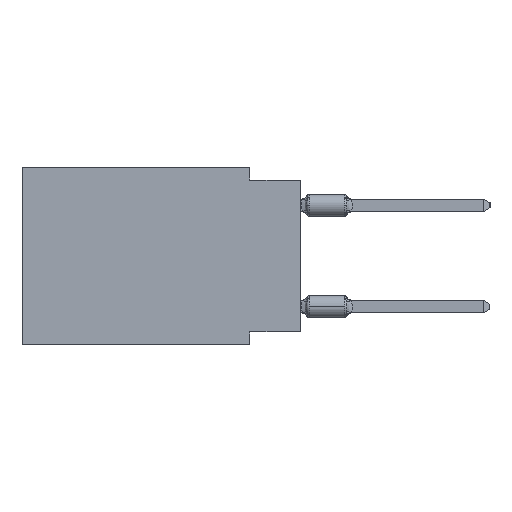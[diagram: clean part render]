
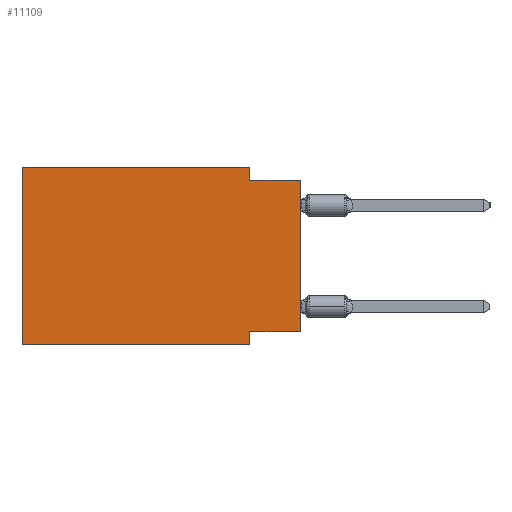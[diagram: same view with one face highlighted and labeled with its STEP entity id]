
A CAD part, left-side view. The second image highlights one B-rep face of the part: STEP entity #11109.
In plain terms, the highlighted planar face has unit normal (-1, 0, 0).
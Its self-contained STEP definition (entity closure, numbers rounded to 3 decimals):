
#362 = EDGE_CURVE ( 'NONE', #3799, #5954, #26076, .T. ) ;
#627 = ORIENTED_EDGE ( 'NONE', *, *, #13560, .T. ) ;
#1425 = LINE ( 'NONE', #3685, #17631 ) ;
#2826 = ORIENTED_EDGE ( 'NONE', *, *, #362, .F. ) ;
#3096 = EDGE_CURVE ( 'NONE', #16999, #22107, #26939, .T. ) ;
#3187 = EDGE_CURVE ( 'NONE', #3863, #16999, #23690, .T. ) ;
#3685 = CARTESIAN_POINT ( 'NONE',  ( 0., 13.97, -8.89 ) ) ;
#3799 = VERTEX_POINT ( 'NONE', #5236 ) ;
#3835 = VECTOR ( 'NONE', #4598, 1000. ) ;
#3863 = VERTEX_POINT ( 'NONE', #5098 ) ;
#4058 = CARTESIAN_POINT ( 'NONE',  ( 0., 13.97, 0. ) ) ;
#4166 = CARTESIAN_POINT ( 'NONE',  ( 0., 0., -8.255 ) ) ;
#4598 = DIRECTION ( 'NONE',  ( 0., 0., 1. ) ) ;
#4613 = VECTOR ( 'NONE', #23969, 1000. ) ;
#4740 = CARTESIAN_POINT ( 'NONE',  ( 0., 0., 0. ) ) ;
#5098 = CARTESIAN_POINT ( 'NONE',  ( 0., 0., -8.255 ) ) ;
#5126 = CARTESIAN_POINT ( 'NONE',  ( 0., 2.54, -8.255 ) ) ;
#5151 = EDGE_CURVE ( 'NONE', #5954, #16354, #18944, .T. ) ;
#5236 = CARTESIAN_POINT ( 'NONE',  ( 0., 2.54, 0. ) ) ;
#5716 = ORIENTED_EDGE ( 'NONE', *, *, #3187, .F. ) ;
#5859 = CARTESIAN_POINT ( 'NONE',  ( 0., 13.97, 0. ) ) ;
#5954 = VERTEX_POINT ( 'NONE', #16780 ) ;
#6368 = EDGE_CURVE ( 'NONE', #6394, #22107, #1425, .T. ) ;
#6394 = VERTEX_POINT ( 'NONE', #14779 ) ;
#6710 = VECTOR ( 'NONE', #27196, 1000. ) ;
#8221 = CARTESIAN_POINT ( 'NONE',  ( 0., 13.97, 0. ) ) ;
#8245 = VECTOR ( 'NONE', #16263, 1000. ) ;
#8878 = CARTESIAN_POINT ( 'NONE',  ( 0., 13.97, 0. ) ) ;
#10136 = ORIENTED_EDGE ( 'NONE', *, *, #18076, .F. ) ;
#10208 = FACE_OUTER_BOUND ( 'NONE', #23736, .T. ) ;
#11109 = ADVANCED_FACE ( 'NONE', ( #10208 ), #14158, .F. ) ;
#11986 = CARTESIAN_POINT ( 'NONE',  ( 0., 0., -0.635 ) ) ;
#12277 = ORIENTED_EDGE ( 'NONE', *, *, #3096, .F. ) ;
#13560 = EDGE_CURVE ( 'NONE', #3863, #16354, #23983, .T. ) ;
#14158 = PLANE ( 'NONE',  #24472 ) ;
#14528 = VECTOR ( 'NONE', #26075, 1000. ) ;
#14779 = CARTESIAN_POINT ( 'NONE',  ( 0., 13.97, -8.89 ) ) ;
#15406 = CARTESIAN_POINT ( 'NONE',  ( 0., 2.54, 0. ) ) ;
#16263 = DIRECTION ( 'NONE',  ( 0., 0., -1. ) ) ;
#16354 = VERTEX_POINT ( 'NONE', #11986 ) ;
#16383 = LINE ( 'NONE', #8221, #6710 ) ;
#16607 = DIRECTION ( 'NONE',  ( 0., -1., 0. ) ) ;
#16708 = LINE ( 'NONE', #4058, #18580 ) ;
#16780 = CARTESIAN_POINT ( 'NONE',  ( 0., 2.54, -0.635 ) ) ;
#16999 = VERTEX_POINT ( 'NONE', #5126 ) ;
#17631 = VECTOR ( 'NONE', #16607, 1000. ) ;
#18076 = EDGE_CURVE ( 'NONE', #6394, #18850, #16708, .T. ) ;
#18369 = CARTESIAN_POINT ( 'NONE',  ( 0., 2.54, -8.89 ) ) ;
#18580 = VECTOR ( 'NONE', #21486, 1000. ) ;
#18850 = VERTEX_POINT ( 'NONE', #8878 ) ;
#18944 = LINE ( 'NONE', #21188, #23857 ) ;
#20095 = ORIENTED_EDGE ( 'NONE', *, *, #6368, .T. ) ;
#20931 = ORIENTED_EDGE ( 'NONE', *, *, #21474, .F. ) ;
#21188 = CARTESIAN_POINT ( 'NONE',  ( 0., 0., -0.635 ) ) ;
#21474 = EDGE_CURVE ( 'NONE', #18850, #3799, #16383, .T. ) ;
#21478 = DIRECTION ( 'NONE',  ( 0., -1., 0. ) ) ;
#21486 = DIRECTION ( 'NONE',  ( 0., 0., 1. ) ) ;
#22107 = VERTEX_POINT ( 'NONE', #24143 ) ;
#22726 = DIRECTION ( 'NONE',  ( 0., 0., -1. ) ) ;
#23189 = ORIENTED_EDGE ( 'NONE', *, *, #5151, .F. ) ;
#23690 = LINE ( 'NONE', #4166, #14528 ) ;
#23736 = EDGE_LOOP ( 'NONE', ( #627, #23189, #2826, #20931, #10136, #20095, #12277, #5716 ) ) ;
#23857 = VECTOR ( 'NONE', #21478, 1000. ) ;
#23969 = DIRECTION ( 'NONE',  ( 0., 0., -1. ) ) ;
#23983 = LINE ( 'NONE', #4740, #3835 ) ;
#24143 = CARTESIAN_POINT ( 'NONE',  ( 0., 2.54, -8.89 ) ) ;
#24472 = AXIS2_PLACEMENT_3D ( 'NONE', #5859, #26932, #22726 ) ;
#26075 = DIRECTION ( 'NONE',  ( 0., 1., 0. ) ) ;
#26076 = LINE ( 'NONE', #15406, #4613 ) ;
#26932 = DIRECTION ( 'NONE',  ( 1., 0., 0. ) ) ;
#26939 = LINE ( 'NONE', #18369, #8245 ) ;
#27196 = DIRECTION ( 'NONE',  ( 0., -1., 0. ) ) ;
